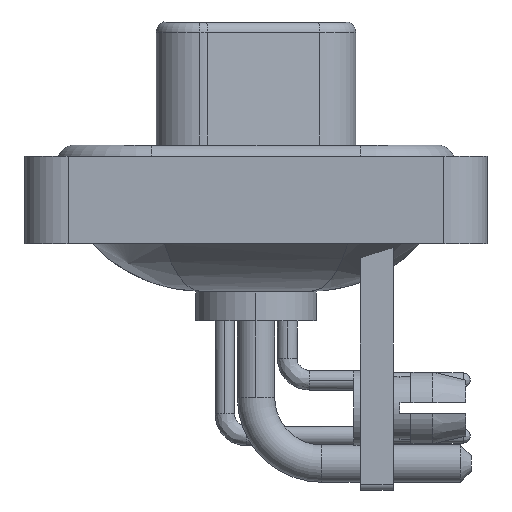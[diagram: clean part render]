
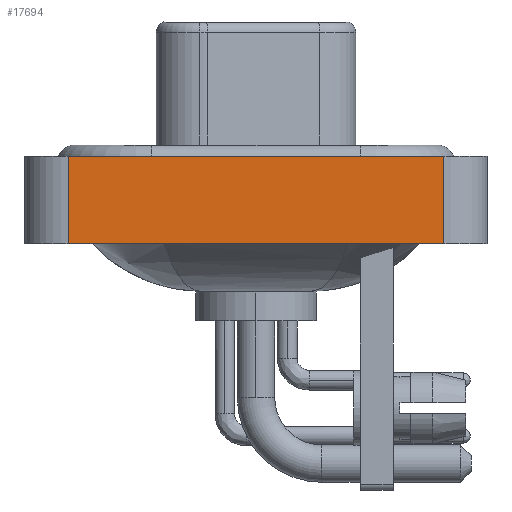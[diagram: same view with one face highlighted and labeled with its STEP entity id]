
A CAD part, left-side view. The second image highlights one B-rep face of the part: STEP entity #17694.
In plain terms, the highlighted planar face has unit normal (-1, 0, 0).
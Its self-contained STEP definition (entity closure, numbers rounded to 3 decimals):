
#155 = VECTOR ( 'NONE', #1100, 1000. ) ;
#1100 = DIRECTION ( 'NONE',  ( 0., -1., 0. ) ) ;
#2680 = VECTOR ( 'NONE', #7954, 1000. ) ;
#2774 = ORIENTED_EDGE ( 'NONE', *, *, #20910, .T. ) ;
#3132 = FACE_OUTER_BOUND ( 'NONE', #13702, .T. ) ;
#3202 = CARTESIAN_POINT ( 'NONE',  ( -7.3, -8.55, 0.4 ) ) ;
#3332 = DIRECTION ( 'NONE',  ( 0., -1., 0. ) ) ;
#4640 = PLANE ( 'NONE',  #11281 ) ;
#5487 = ORIENTED_EDGE ( 'NONE', *, *, #14634, .F. ) ;
#7610 = CARTESIAN_POINT ( 'NONE',  ( -7.3, -8.55, -3.6 ) ) ;
#7954 = DIRECTION ( 'NONE',  ( 0., 0., 1. ) ) ;
#8551 = VECTOR ( 'NONE', #26453, 1000. ) ;
#10148 = CARTESIAN_POINT ( 'NONE',  ( -7.3, -8.55, 0.4 ) ) ;
#10377 = ORIENTED_EDGE ( 'NONE', *, *, #11081, .T. ) ;
#10711 = VERTEX_POINT ( 'NONE', #17263 ) ;
#11081 = EDGE_CURVE ( 'NONE', #10711, #19041, #18237, .T. ) ;
#11281 = AXIS2_PLACEMENT_3D ( 'NONE', #7610, #24396, #19770 ) ;
#11430 = VECTOR ( 'NONE', #3332, 1000. ) ;
#13702 = EDGE_LOOP ( 'NONE', ( #2774, #5487, #24442, #10377 ) ) ;
#14090 = LINE ( 'NONE', #22834, #2680 ) ;
#14634 = EDGE_CURVE ( 'NONE', #26734, #20895, #16116, .T. ) ;
#15675 = CARTESIAN_POINT ( 'NONE',  ( -7.3, 8.55, -3.6 ) ) ;
#15745 = CARTESIAN_POINT ( 'NONE',  ( -7.3, -8.55, -3.6 ) ) ;
#16116 = LINE ( 'NONE', #3202, #11430 ) ;
#17263 = CARTESIAN_POINT ( 'NONE',  ( -7.3, 8.55, -3.6 ) ) ;
#17694 = ADVANCED_FACE ( 'NONE', ( #3132 ), #4640, .T. ) ;
#18237 = LINE ( 'NONE', #22341, #155 ) ;
#19041 = VERTEX_POINT ( 'NONE', #15745 ) ;
#19770 = DIRECTION ( 'NONE',  ( 0., 0., 1. ) ) ;
#19788 = LINE ( 'NONE', #15675, #8551 ) ;
#20169 = CARTESIAN_POINT ( 'NONE',  ( -7.3, 8.55, 0.4 ) ) ;
#20895 = VERTEX_POINT ( 'NONE', #10148 ) ;
#20910 = EDGE_CURVE ( 'NONE', #19041, #20895, #14090, .T. ) ;
#22341 = CARTESIAN_POINT ( 'NONE',  ( -7.3, -8.55, -3.6 ) ) ;
#22834 = CARTESIAN_POINT ( 'NONE',  ( -7.3, -8.55, -3.6 ) ) ;
#24396 = DIRECTION ( 'NONE',  ( -1., 0., 0. ) ) ;
#24442 = ORIENTED_EDGE ( 'NONE', *, *, #25470, .F. ) ;
#25470 = EDGE_CURVE ( 'NONE', #10711, #26734, #19788, .T. ) ;
#26453 = DIRECTION ( 'NONE',  ( 0., 0., 1. ) ) ;
#26734 = VERTEX_POINT ( 'NONE', #20169 ) ;
